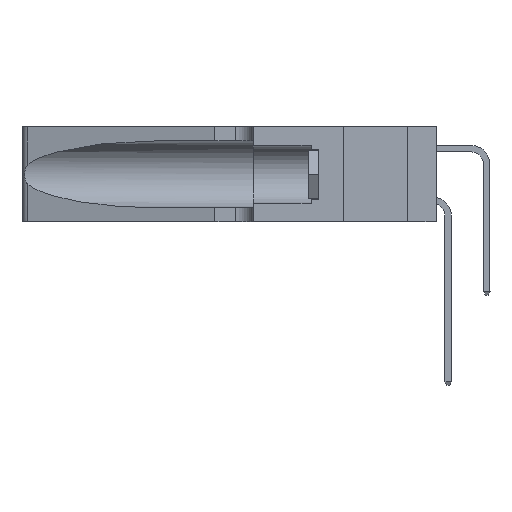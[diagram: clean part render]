
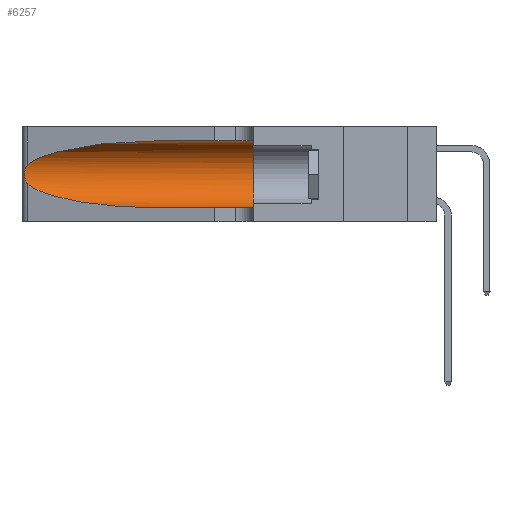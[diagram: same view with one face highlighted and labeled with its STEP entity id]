
A CAD part, left-side view. The second image highlights one B-rep face of the part: STEP entity #6257.
In plain terms, the highlighted cylindrical face has radius 3.308 mm (diameter 6.617 mm), a partial arc.
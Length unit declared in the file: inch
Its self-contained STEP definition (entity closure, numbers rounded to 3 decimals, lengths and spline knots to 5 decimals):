
#79 = AXIS2_PLACEMENT_3D ( 'NONE', #9898, #1101, #10031 ) ;
#604 = CYLINDRICAL_SURFACE ( 'NONE', #79, 0.13025 ) ;
#1101 = DIRECTION ( 'NONE',  ( 0., -1., 0. ) ) ;
#1652 = CIRCLE ( 'NONE', #4745, 0.13025 ) ;
#3211 = CARTESIAN_POINT ( 'NONE',  ( 0.1305, 0.72297, 0.31525 ) ) ;
#3249 =( BOUNDED_CURVE ( )  B_SPLINE_CURVE ( 3, ( #32645, #3466, #6466, #9455 ),
 .UNSPECIFIED., .F., .T. ) 
 B_SPLINE_CURVE_WITH_KNOTS ( ( 4, 4 ),
 ( 1.5708, 2.84003 ),
 .UNSPECIFIED. ) 
 CURVE ( )  GEOMETRIC_REPRESENTATION_ITEM ( )  RATIONAL_B_SPLINE_CURVE ( ( 1., 0.87, 0.87, 1. ) ) 
 REPRESENTATION_ITEM ( '' )  );
#3466 = CARTESIAN_POINT ( 'NONE',  ( 0.18966, 0.96281, 0.31525 ) ) ;
#4153 = DIRECTION ( 'NONE',  ( 0., -1., 0. ) ) ;
#4596 = CARTESIAN_POINT ( 'NONE',  ( 0.1305, 1.61858, 0.31525 ) ) ;
#4745 = AXIS2_PLACEMENT_3D ( 'NONE', #32027, #8173, #5451 ) ;
#5451 = DIRECTION ( 'NONE',  ( 0., 0., 1. ) ) ;
#6257 = ADVANCED_FACE ( 'NONE', ( #31536 ), #604, .F. ) ;
#6466 = CARTESIAN_POINT ( 'NONE',  ( 0.2373, 1.15595, 0.28018 ) ) ;
#7437 = CARTESIAN_POINT ( 'NONE',  ( 0.1305, 0.72297, 0.05475 ) ) ;
#7947 = LINE ( 'NONE', #4596, #25971 ) ;
#8071 = CARTESIAN_POINT ( 'NONE',  ( 0.25856, 1.23593, 0.16098 ) ) ;
#8173 = DIRECTION ( 'NONE',  ( 0., 1., 0. ) ) ;
#9455 = CARTESIAN_POINT ( 'NONE',  ( 0.25487, 1.22718, 0.22369 ) ) ;
#9887 = VERTEX_POINT ( 'NONE', #15720 ) ;
#9898 = CARTESIAN_POINT ( 'NONE',  ( 0.1305, 1.61858, 0.185 ) ) ;
#10031 = DIRECTION ( 'NONE',  ( 0., 0., -1. ) ) ;
#10046 = DIRECTION ( 'NONE',  ( 0., -1., 0. ) ) ;
#10094 = CARTESIAN_POINT ( 'NONE',  ( 0.25487, 1.22718, 0.22369 ) ) ;
#10825 = CARTESIAN_POINT ( 'NONE',  ( 0.25555, 1.22994, 0.2215 ) ) ;
#11292 = ORIENTED_EDGE ( 'NONE', *, *, #15750, .T. ) ;
#14066 = CARTESIAN_POINT ( 'NONE',  ( 0.26017, 1.23833, 0.17102 ) ) ;
#15424 = EDGE_LOOP ( 'NONE', ( #11292, #33996, #21235, #32705, #33844, #32728 ) ) ;
#15720 = CARTESIAN_POINT ( 'NONE',  ( 0.1305, 0.72297, 0.05475 ) ) ;
#15750 = EDGE_CURVE ( 'NONE', #17120, #22446, #3249, .T. ) ;
#16019 = EDGE_CURVE ( 'NONE', #31138, #9887, #17509, .T. ) ;
#17017 = CARTESIAN_POINT ( 'NONE',  ( 0.26018, 1.23835, 0.19895 ) ) ;
#17120 = VERTEX_POINT ( 'NONE', #3211 ) ;
#17130 = CARTESIAN_POINT ( 'NONE',  ( 0.25555, 1.22993, 0.14849 ) ) ;
#17509 =( BOUNDED_CURVE ( )  B_SPLINE_CURVE ( 3, ( #27975, #33861, #19319, #7437 ),
 .UNSPECIFIED., .F., .T. ) 
 B_SPLINE_CURVE_WITH_KNOTS ( ( 4, 4 ),
 ( 3.44316, 4.71239 ),
 .UNSPECIFIED. ) 
 CURVE ( )  GEOMETRIC_REPRESENTATION_ITEM ( )  RATIONAL_B_SPLINE_CURVE ( ( 1., 0.87, 0.87, 1. ) ) 
 REPRESENTATION_ITEM ( '' )  );
#19112 = EDGE_CURVE ( 'NONE', #24673, #30444, #1652, .T. ) ;
#19319 = CARTESIAN_POINT ( 'NONE',  ( 0.18966, 0.96281, 0.05475 ) ) ;
#20238 = CARTESIAN_POINT ( 'NONE',  ( 0.25639, 1.23186, 0.15144 ) ) ;
#21235 = ORIENTED_EDGE ( 'NONE', *, *, #16019, .T. ) ;
#22003 = EDGE_CURVE ( 'NONE', #17120, #24673, #7947, .T. ) ;
#22446 = VERTEX_POINT ( 'NONE', #10094 ) ;
#22766 = CARTESIAN_POINT ( 'NONE',  ( 0.25487, 1.22718, 0.14631 ) ) ;
#23060 = CARTESIAN_POINT ( 'NONE',  ( 0.25487, 1.22718, 0.14631 ) ) ;
#24673 = VERTEX_POINT ( 'NONE', #27874 ) ;
#25777 = CARTESIAN_POINT ( 'NONE',  ( 0.25854, 1.2359, 0.20912 ) ) ;
#25971 = VECTOR ( 'NONE', #10046, 39.37008 ) ;
#26037 = CARTESIAN_POINT ( 'NONE',  ( 0.25639, 1.23184, 0.21858 ) ) ;
#26876 = LINE ( 'NONE', #27682, #33758 ) ;
#27682 = CARTESIAN_POINT ( 'NONE',  ( 0.1305, 1.61858, 0.05475 ) ) ;
#27874 = CARTESIAN_POINT ( 'NONE',  ( 0.1305, 0.35, 0.31525 ) ) ;
#27975 = CARTESIAN_POINT ( 'NONE',  ( 0.25487, 1.22718, 0.14631 ) ) ;
#28560 = EDGE_CURVE ( 'NONE', #22446, #31138, #32366, .T. ) ;
#28629 = CARTESIAN_POINT ( 'NONE',  ( 0.26075, 1.23896, 0.19203 ) ) ;
#28635 = CARTESIAN_POINT ( 'NONE',  ( 0.1305, 0.35, 0.05475 ) ) ;
#30444 = VERTEX_POINT ( 'NONE', #28635 ) ;
#31138 = VERTEX_POINT ( 'NONE', #22766 ) ;
#31422 = CARTESIAN_POINT ( 'NONE',  ( 0.25787, 1.23484, 0.2124 ) ) ;
#31536 = FACE_OUTER_BOUND ( 'NONE', #15424, .T. ) ;
#32027 = CARTESIAN_POINT ( 'NONE',  ( 0.1305, 0.35, 0.185 ) ) ;
#32366 = B_SPLINE_CURVE_WITH_KNOTS ( 'NONE', 3,
 ( #37356, #10825, #26037, #31422, #25777, #17017, #28629, #34514, #14066, #8071, #37737, #20238, #17130, #23060 ),
 .UNSPECIFIED., .F., .F.,
 ( 4, 2, 2, 2, 2, 2, 4 ),
 ( 0., 0.00027, 0.00053, 0.00107, 0.0016, 0.00187, 0.00214 ),
 .UNSPECIFIED. ) ;
#32645 = CARTESIAN_POINT ( 'NONE',  ( 0.1305, 0.72297, 0.31525 ) ) ;
#32705 = ORIENTED_EDGE ( 'NONE', *, *, #35370, .T. ) ;
#32728 = ORIENTED_EDGE ( 'NONE', *, *, #22003, .F. ) ;
#33758 = VECTOR ( 'NONE', #4153, 39.37008 ) ;
#33844 = ORIENTED_EDGE ( 'NONE', *, *, #19112, .F. ) ;
#33861 = CARTESIAN_POINT ( 'NONE',  ( 0.2373, 1.15595, 0.08982 ) ) ;
#33996 = ORIENTED_EDGE ( 'NONE', *, *, #28560, .T. ) ;
#34514 = CARTESIAN_POINT ( 'NONE',  ( 0.26075, 1.23896, 0.178 ) ) ;
#35370 = EDGE_CURVE ( 'NONE', #9887, #30444, #26876, .T. ) ;
#37356 = CARTESIAN_POINT ( 'NONE',  ( 0.25487, 1.22718, 0.22369 ) ) ;
#37737 = CARTESIAN_POINT ( 'NONE',  ( 0.25789, 1.23486, 0.15765 ) ) ;
